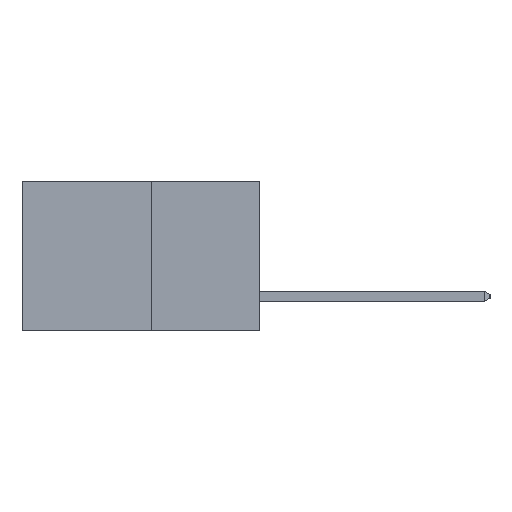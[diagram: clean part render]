
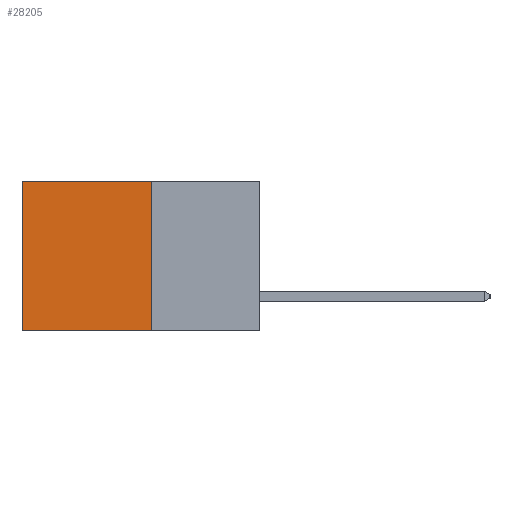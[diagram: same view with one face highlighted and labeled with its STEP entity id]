
A CAD part, left-side view. The second image highlights one B-rep face of the part: STEP entity #28205.
In plain terms, the highlighted planar face has unit normal (-1, 0, 0).
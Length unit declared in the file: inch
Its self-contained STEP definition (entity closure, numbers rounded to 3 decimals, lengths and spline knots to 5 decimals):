
#645 = VECTOR ( 'NONE', #16142, 39.37008 ) ;
#857 = PLANE ( 'NONE',  #8698 ) ;
#945 = DIRECTION ( 'NONE',  ( 0., 0., -1. ) ) ;
#3159 = VERTEX_POINT ( 'NONE', #15412 ) ;
#3965 = VECTOR ( 'NONE', #11831, 39.37008 ) ;
#5194 = CARTESIAN_POINT ( 'NONE',  ( 0.277, 0.27, -0.37 ) ) ;
#6900 = EDGE_CURVE ( 'NONE', #3159, #11186, #15913, .T. ) ;
#7426 = LINE ( 'NONE', #12564, #12535 ) ;
#8698 = AXIS2_PLACEMENT_3D ( 'NONE', #20580, #14000, #945 ) ;
#10261 = CARTESIAN_POINT ( 'NONE',  ( 0.277, 0.27, -0.37 ) ) ;
#10327 = VERTEX_POINT ( 'NONE', #10261 ) ;
#10745 = EDGE_CURVE ( 'NONE', #10327, #11186, #23901, .T. ) ;
#11186 = VERTEX_POINT ( 'NONE', #21954 ) ;
#11831 = DIRECTION ( 'NONE',  ( 0., 1., 0. ) ) ;
#12535 = VECTOR ( 'NONE', #14783, 39.37008 ) ;
#12564 = CARTESIAN_POINT ( 'NONE',  ( 0.277, 0.27, -0.37 ) ) ;
#14000 = DIRECTION ( 'NONE',  ( 1., 0., 0. ) ) ;
#14187 = DIRECTION ( 'NONE',  ( 0., 0., -1. ) ) ;
#14265 = ORIENTED_EDGE ( 'NONE', *, *, #17385, .F. ) ;
#14783 = DIRECTION ( 'NONE',  ( 0., 0., -1. ) ) ;
#15412 = CARTESIAN_POINT ( 'NONE',  ( 0.277, 0.59, 0. ) ) ;
#15913 = LINE ( 'NONE', #25119, #21064 ) ;
#16142 = DIRECTION ( 'NONE',  ( 0., 1., 0. ) ) ;
#16234 = ORIENTED_EDGE ( 'NONE', *, *, #6900, .T. ) ;
#17385 = EDGE_CURVE ( 'NONE', #18625, #10327, #7426, .T. ) ;
#18625 = VERTEX_POINT ( 'NONE', #21528 ) ;
#19595 = EDGE_LOOP ( 'NONE', ( #16234, #24350, #14265, #26326 ) ) ;
#20580 = CARTESIAN_POINT ( 'NONE',  ( 0.277, 0.27, -0.37 ) ) ;
#20616 = CARTESIAN_POINT ( 'NONE',  ( 0.277, 0.27, 0. ) ) ;
#21064 = VECTOR ( 'NONE', #14187, 39.37008 ) ;
#21472 = LINE ( 'NONE', #20616, #3965 ) ;
#21528 = CARTESIAN_POINT ( 'NONE',  ( 0.277, 0.27, 0. ) ) ;
#21954 = CARTESIAN_POINT ( 'NONE',  ( 0.277, 0.59, -0.37 ) ) ;
#23488 = EDGE_CURVE ( 'NONE', #18625, #3159, #21472, .T. ) ;
#23812 = FACE_OUTER_BOUND ( 'NONE', #19595, .T. ) ;
#23901 = LINE ( 'NONE', #5194, #645 ) ;
#24350 = ORIENTED_EDGE ( 'NONE', *, *, #10745, .F. ) ;
#25119 = CARTESIAN_POINT ( 'NONE',  ( 0.277, 0.59, -0.37 ) ) ;
#26326 = ORIENTED_EDGE ( 'NONE', *, *, #23488, .T. ) ;
#28205 = ADVANCED_FACE ( 'NONE', ( #23812 ), #857, .F. ) ;
